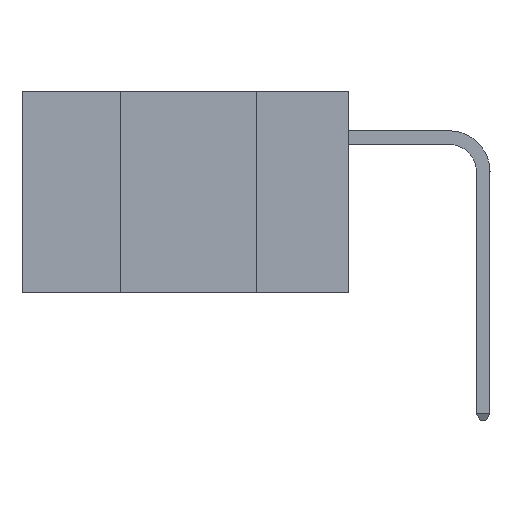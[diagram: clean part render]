
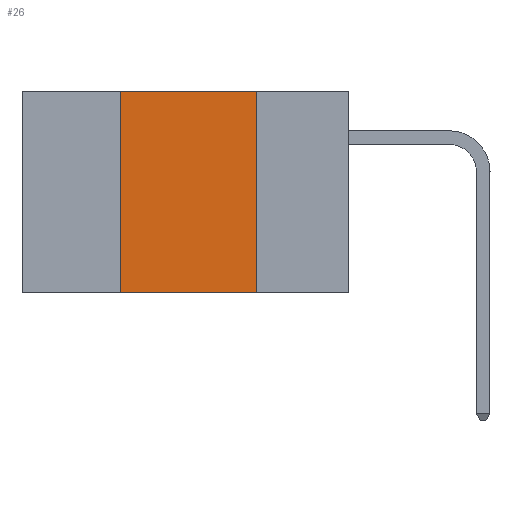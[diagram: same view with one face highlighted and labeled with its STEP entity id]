
A CAD part, left-side view. The second image highlights one B-rep face of the part: STEP entity #26.
In plain terms, the highlighted planar face has unit normal (-1, 0, 0).
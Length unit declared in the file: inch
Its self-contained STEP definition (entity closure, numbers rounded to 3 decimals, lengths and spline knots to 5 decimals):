
#26 = ADVANCED_FACE ( 'NONE', ( #17929 ), #16906, .F. ) ;
#42 = CARTESIAN_POINT ( 'NONE',  ( 0., 0.42, -0.37 ) ) ;
#560 = LINE ( 'NONE', #15272, #12138 ) ;
#975 = EDGE_CURVE ( 'NONE', #2526, #3250, #8075, .T. ) ;
#1720 = AXIS2_PLACEMENT_3D ( 'NONE', #16872, #15241, #12726 ) ;
#1782 = CARTESIAN_POINT ( 'NONE',  ( 0., 0.17, 0. ) ) ;
#1982 = VECTOR ( 'NONE', #9403, 39.37008 ) ;
#2480 = CARTESIAN_POINT ( 'NONE',  ( 0., 0.17, 0. ) ) ;
#2526 = VERTEX_POINT ( 'NONE', #42 ) ;
#3250 = VERTEX_POINT ( 'NONE', #16521 ) ;
#3616 = VECTOR ( 'NONE', #16954, 39.37008 ) ;
#6057 = LINE ( 'NONE', #16814, #1982 ) ;
#6203 = LINE ( 'NONE', #1782, #11573 ) ;
#6795 = EDGE_CURVE ( 'NONE', #3250, #8832, #6057, .T. ) ;
#7826 = DIRECTION ( 'NONE',  ( 0., 0., -1. ) ) ;
#8061 = CARTESIAN_POINT ( 'NONE',  ( 0., 0.17, -0.37 ) ) ;
#8075 = LINE ( 'NONE', #16821, #3616 ) ;
#8832 = VERTEX_POINT ( 'NONE', #2480 ) ;
#9403 = DIRECTION ( 'NONE',  ( 0., -1., 0. ) ) ;
#9734 = EDGE_CURVE ( 'NONE', #8832, #10477, #6203, .T. ) ;
#10477 = VERTEX_POINT ( 'NONE', #8061 ) ;
#10661 = ORIENTED_EDGE ( 'NONE', *, *, #975, .F. ) ;
#11573 = VECTOR ( 'NONE', #7826, 39.37008 ) ;
#12138 = VECTOR ( 'NONE', #16736, 39.37008 ) ;
#12726 = DIRECTION ( 'NONE',  ( 0., 0., -1. ) ) ;
#13715 = ORIENTED_EDGE ( 'NONE', *, *, #9734, .F. ) ;
#14665 = ORIENTED_EDGE ( 'NONE', *, *, #15523, .T. ) ;
#15241 = DIRECTION ( 'NONE',  ( 1., 0., 0. ) ) ;
#15272 = CARTESIAN_POINT ( 'NONE',  ( 0., 0.6, -0.37 ) ) ;
#15523 = EDGE_CURVE ( 'NONE', #2526, #10477, #560, .T. ) ;
#15735 = EDGE_LOOP ( 'NONE', ( #13715, #17667, #10661, #14665 ) ) ;
#16521 = CARTESIAN_POINT ( 'NONE',  ( 0., 0.42, 0. ) ) ;
#16736 = DIRECTION ( 'NONE',  ( 0., -1., 0. ) ) ;
#16814 = CARTESIAN_POINT ( 'NONE',  ( 0., 0.6, 0. ) ) ;
#16821 = CARTESIAN_POINT ( 'NONE',  ( 0., 0.42, 0. ) ) ;
#16872 = CARTESIAN_POINT ( 'NONE',  ( 0., 0.6, 0. ) ) ;
#16906 = PLANE ( 'NONE',  #1720 ) ;
#16954 = DIRECTION ( 'NONE',  ( 0., 0., 1. ) ) ;
#17667 = ORIENTED_EDGE ( 'NONE', *, *, #6795, .F. ) ;
#17929 = FACE_OUTER_BOUND ( 'NONE', #15735, .T. ) ;
